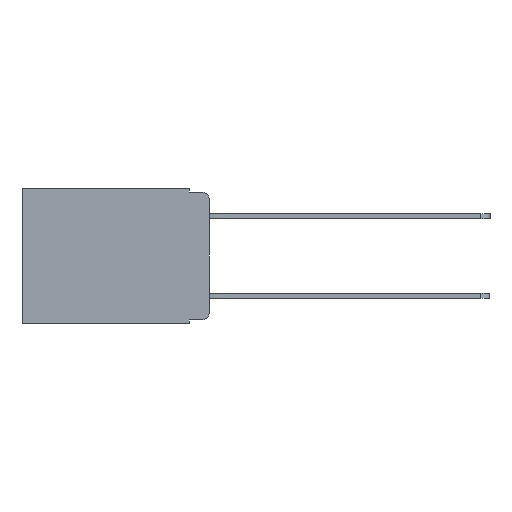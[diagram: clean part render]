
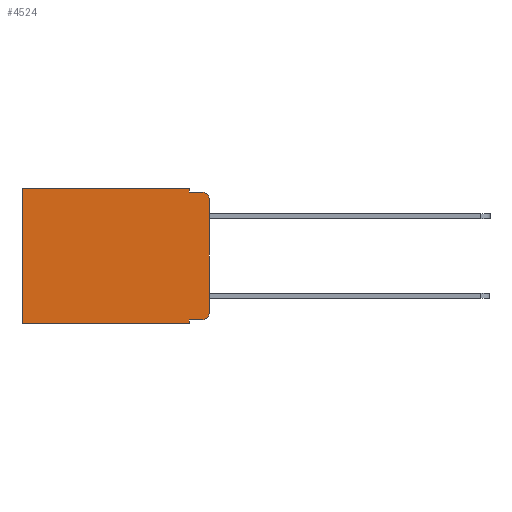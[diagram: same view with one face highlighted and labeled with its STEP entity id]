
A CAD part, left-side view. The second image highlights one B-rep face of the part: STEP entity #4524.
In plain terms, the highlighted planar face has unit normal (-1, 0, 0).
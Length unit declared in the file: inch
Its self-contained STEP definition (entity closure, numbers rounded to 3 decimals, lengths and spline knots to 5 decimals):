
#184 = CARTESIAN_POINT ( 'NONE',  ( 0.298, 0., 0. ) ) ;
#301 = VECTOR ( 'NONE', #9716, 39.37008 ) ;
#372 = VECTOR ( 'NONE', #3048, 39.37008 ) ;
#517 = VERTEX_POINT ( 'NONE', #3786 ) ;
#697 = DIRECTION ( 'NONE',  ( -1., 0., 0. ) ) ;
#1116 = LINE ( 'NONE', #2995, #372 ) ;
#1307 = VERTEX_POINT ( 'NONE', #1692 ) ;
#1624 = ORIENTED_EDGE ( 'NONE', *, *, #5150, .F. ) ;
#1692 = CARTESIAN_POINT ( 'NONE',  ( 0.298, 0.051, 0. ) ) ;
#1774 = LINE ( 'NONE', #11189, #8724 ) ;
#1775 = CARTESIAN_POINT ( 'NONE',  ( 0.298, 0.473, -0.343 ) ) ;
#1987 = VERTEX_POINT ( 'NONE', #8827 ) ;
#2350 = CARTESIAN_POINT ( 'NONE',  ( 0.298, 0.02, -0.313 ) ) ;
#2413 = AXIS2_PLACEMENT_3D ( 'NONE', #6679, #697, #7571 ) ;
#2697 = CARTESIAN_POINT ( 'NONE',  ( 0.298, 0.051, -0.333 ) ) ;
#2995 = CARTESIAN_POINT ( 'NONE',  ( 0.298, 0., 0. ) ) ;
#3048 = DIRECTION ( 'NONE',  ( 0., 0., -1. ) ) ;
#3405 = DIRECTION ( 'NONE',  ( 0., 0., -1. ) ) ;
#3484 = DIRECTION ( 'NONE',  ( 0., 1., 0. ) ) ;
#3597 = DIRECTION ( 'NONE',  ( 0., 0., -1. ) ) ;
#3786 = CARTESIAN_POINT ( 'NONE',  ( 0.298, 0.051, -0.01 ) ) ;
#4048 = ORIENTED_EDGE ( 'NONE', *, *, #10774, .T. ) ;
#4208 = CARTESIAN_POINT ( 'NONE',  ( 0.298, 0., -0.03 ) ) ;
#4383 = EDGE_CURVE ( 'NONE', #1307, #517, #9916, .T. ) ;
#4419 = ORIENTED_EDGE ( 'NONE', *, *, #5277, .F. ) ;
#4485 = ORIENTED_EDGE ( 'NONE', *, *, #7294, .F. ) ;
#4524 = ADVANCED_FACE ( 'NONE', ( #10799 ), #10880, .F. ) ;
#4576 = EDGE_CURVE ( 'NONE', #5835, #7681, #8307, .T. ) ;
#4597 = ORIENTED_EDGE ( 'NONE', *, *, #5196, .T. ) ;
#4782 = ORIENTED_EDGE ( 'NONE', *, *, #5813, .T. ) ;
#5028 = ORIENTED_EDGE ( 'NONE', *, *, #4383, .F. ) ;
#5033 = CIRCLE ( 'NONE', #2413, 0.02 ) ;
#5086 = VERTEX_POINT ( 'NONE', #8605 ) ;
#5150 = EDGE_CURVE ( 'NONE', #8463, #5835, #1774, .T. ) ;
#5196 = EDGE_CURVE ( 'NONE', #5553, #7681, #6055, .T. ) ;
#5210 = VECTOR ( 'NONE', #3597, 39.37008 ) ;
#5277 = EDGE_CURVE ( 'NONE', #517, #10555, #8143, .T. ) ;
#5284 = CARTESIAN_POINT ( 'NONE',  ( 0.298, 0.051, -0.333 ) ) ;
#5290 = EDGE_CURVE ( 'NONE', #5086, #1987, #10161, .T. ) ;
#5307 = EDGE_CURVE ( 'NONE', #8463, #5086, #5472, .T. ) ;
#5472 = LINE ( 'NONE', #5284, #301 ) ;
#5553 = VERTEX_POINT ( 'NONE', #11550 ) ;
#5780 = CARTESIAN_POINT ( 'NONE',  ( 0.298, 0.051, -0.343 ) ) ;
#5784 = ORIENTED_EDGE ( 'NONE', *, *, #5307, .T. ) ;
#5813 = EDGE_CURVE ( 'NONE', #9782, #10555, #5033, .T. ) ;
#5835 = VERTEX_POINT ( 'NONE', #5780 ) ;
#6055 = LINE ( 'NONE', #11267, #10405 ) ;
#6592 = LINE ( 'NONE', #184, #8698 ) ;
#6679 = CARTESIAN_POINT ( 'NONE',  ( 0.298, 0.02, -0.03 ) ) ;
#6802 = ORIENTED_EDGE ( 'NONE', *, *, #4576, .F. ) ;
#6971 = DIRECTION ( 'NONE',  ( 0., 0., -1. ) ) ;
#7294 = EDGE_CURVE ( 'NONE', #9782, #1987, #1116, .T. ) ;
#7571 = DIRECTION ( 'NONE',  ( 0., 0., -1. ) ) ;
#7681 = VERTEX_POINT ( 'NONE', #1775 ) ;
#7860 = VECTOR ( 'NONE', #7907, 39.37008 ) ;
#7907 = DIRECTION ( 'NONE',  ( 0., -1., 0. ) ) ;
#8143 = LINE ( 'NONE', #9674, #7860 ) ;
#8307 = LINE ( 'NONE', #9138, #10301 ) ;
#8463 = VERTEX_POINT ( 'NONE', #2697 ) ;
#8605 = CARTESIAN_POINT ( 'NONE',  ( 0.298, 0.02, -0.333 ) ) ;
#8658 = CARTESIAN_POINT ( 'NONE',  ( 0.298, 0.02, -0.01 ) ) ;
#8698 = VECTOR ( 'NONE', #3484, 39.37008 ) ;
#8724 = VECTOR ( 'NONE', #9581, 39.37008 ) ;
#8827 = CARTESIAN_POINT ( 'NONE',  ( 0.298, 0., -0.313 ) ) ;
#8858 = DIRECTION ( 'NONE',  ( -1., 0., 0. ) ) ;
#9138 = CARTESIAN_POINT ( 'NONE',  ( 0.298, 0., -0.343 ) ) ;
#9152 = DIRECTION ( 'NONE',  ( 0., 1., 0. ) ) ;
#9454 = ORIENTED_EDGE ( 'NONE', *, *, #5290, .T. ) ;
#9581 = DIRECTION ( 'NONE',  ( 0., 0., -1. ) ) ;
#9674 = CARTESIAN_POINT ( 'NONE',  ( 0.298, 0.051, -0.01 ) ) ;
#9716 = DIRECTION ( 'NONE',  ( 0., -1., 0. ) ) ;
#9782 = VERTEX_POINT ( 'NONE', #4208 ) ;
#9893 = EDGE_LOOP ( 'NONE', ( #4485, #4782, #4419, #5028, #4048, #4597, #6802, #1624, #5784, #9454 ) ) ;
#9916 = LINE ( 'NONE', #10527, #5210 ) ;
#10026 = CARTESIAN_POINT ( 'NONE',  ( 0.298, 0., 0. ) ) ;
#10161 = CIRCLE ( 'NONE', #12076, 0.02 ) ;
#10301 = VECTOR ( 'NONE', #9152, 39.37008 ) ;
#10405 = VECTOR ( 'NONE', #6971, 39.37008 ) ;
#10527 = CARTESIAN_POINT ( 'NONE',  ( 0.298, 0.051, 0. ) ) ;
#10555 = VERTEX_POINT ( 'NONE', #8658 ) ;
#10774 = EDGE_CURVE ( 'NONE', #1307, #5553, #6592, .T. ) ;
#10799 = FACE_OUTER_BOUND ( 'NONE', #9893, .T. ) ;
#10880 = PLANE ( 'NONE',  #11577 ) ;
#11189 = CARTESIAN_POINT ( 'NONE',  ( 0.298, 0.051, 0. ) ) ;
#11267 = CARTESIAN_POINT ( 'NONE',  ( 0.298, 0.473, 0. ) ) ;
#11466 = DIRECTION ( 'NONE',  ( 0., 0., -1. ) ) ;
#11475 = DIRECTION ( 'NONE',  ( 1., 0., 0. ) ) ;
#11550 = CARTESIAN_POINT ( 'NONE',  ( 0.298, 0.473, 0. ) ) ;
#11577 = AXIS2_PLACEMENT_3D ( 'NONE', #10026, #11475, #11466 ) ;
#12076 = AXIS2_PLACEMENT_3D ( 'NONE', #2350, #8858, #3405 ) ;
